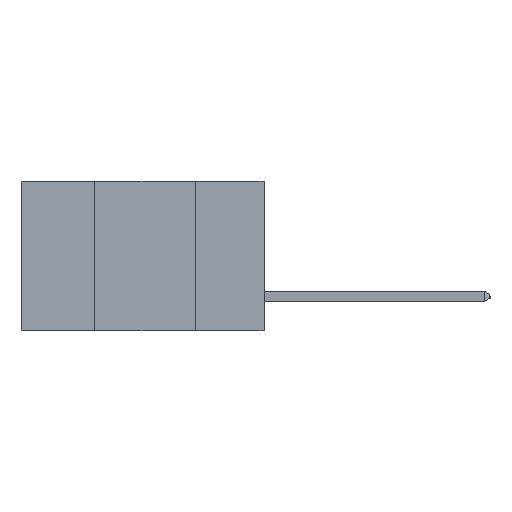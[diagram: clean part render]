
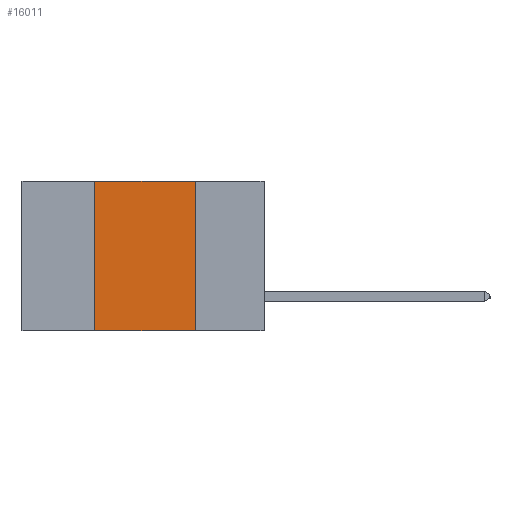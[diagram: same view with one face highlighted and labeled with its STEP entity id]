
A CAD part, left-side view. The second image highlights one B-rep face of the part: STEP entity #16011.
In plain terms, the highlighted planar face has unit normal (-1, 0, 0).
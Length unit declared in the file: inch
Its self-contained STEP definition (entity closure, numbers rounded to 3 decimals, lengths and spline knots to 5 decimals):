
#528 = VERTEX_POINT ( 'NONE', #7414 ) ;
#1300 = VECTOR ( 'NONE', #2792, 39.37008 ) ;
#2302 = CARTESIAN_POINT ( 'NONE',  ( 0., 0.17, -0.37 ) ) ;
#2792 = DIRECTION ( 'NONE',  ( 0., 0., -1. ) ) ;
#3299 = CARTESIAN_POINT ( 'NONE',  ( 0., 0.6, 0. ) ) ;
#4230 = LINE ( 'NONE', #9954, #7280 ) ;
#4385 = VERTEX_POINT ( 'NONE', #16420 ) ;
#4729 = DIRECTION ( 'NONE',  ( 0., 0., -1. ) ) ;
#4787 = CARTESIAN_POINT ( 'NONE',  ( 0., 0.42, 0. ) ) ;
#5479 = EDGE_CURVE ( 'NONE', #528, #14911, #15991, .T. ) ;
#6102 = VECTOR ( 'NONE', #11981, 39.37008 ) ;
#6821 = ORIENTED_EDGE ( 'NONE', *, *, #8893, .F. ) ;
#7280 = VECTOR ( 'NONE', #7431, 39.37008 ) ;
#7414 = CARTESIAN_POINT ( 'NONE',  ( 0., 0.42, -0.37 ) ) ;
#7431 = DIRECTION ( 'NONE',  ( 0., -1., 0. ) ) ;
#7847 = VERTEX_POINT ( 'NONE', #4787 ) ;
#7887 = EDGE_CURVE ( 'NONE', #7847, #4385, #4230, .T. ) ;
#8520 = PLANE ( 'NONE',  #12859 ) ;
#8570 = ORIENTED_EDGE ( 'NONE', *, *, #14144, .F. ) ;
#8893 = EDGE_CURVE ( 'NONE', #528, #7847, #12796, .T. ) ;
#9205 = CARTESIAN_POINT ( 'NONE',  ( 0., 0.17, 0. ) ) ;
#9954 = CARTESIAN_POINT ( 'NONE',  ( 0., 0.6, 0. ) ) ;
#11876 = EDGE_LOOP ( 'NONE', ( #8570, #12718, #6821, #13508 ) ) ;
#11937 = CARTESIAN_POINT ( 'NONE',  ( 0., 0.6, -0.37 ) ) ;
#11981 = DIRECTION ( 'NONE',  ( 0., 0., 1. ) ) ;
#12335 = DIRECTION ( 'NONE',  ( 1., 0., 0. ) ) ;
#12718 = ORIENTED_EDGE ( 'NONE', *, *, #7887, .F. ) ;
#12796 = LINE ( 'NONE', #15602, #6102 ) ;
#12859 = AXIS2_PLACEMENT_3D ( 'NONE', #3299, #12335, #4729 ) ;
#13191 = DIRECTION ( 'NONE',  ( 0., -1., 0. ) ) ;
#13508 = ORIENTED_EDGE ( 'NONE', *, *, #5479, .T. ) ;
#13575 = FACE_OUTER_BOUND ( 'NONE', #11876, .T. ) ;
#14144 = EDGE_CURVE ( 'NONE', #4385, #14911, #14949, .T. ) ;
#14911 = VERTEX_POINT ( 'NONE', #2302 ) ;
#14949 = LINE ( 'NONE', #9205, #1300 ) ;
#15602 = CARTESIAN_POINT ( 'NONE',  ( 0., 0.42, 0. ) ) ;
#15614 = VECTOR ( 'NONE', #13191, 39.37008 ) ;
#15991 = LINE ( 'NONE', #11937, #15614 ) ;
#16011 = ADVANCED_FACE ( 'NONE', ( #13575 ), #8520, .F. ) ;
#16420 = CARTESIAN_POINT ( 'NONE',  ( 0., 0.17, 0. ) ) ;
